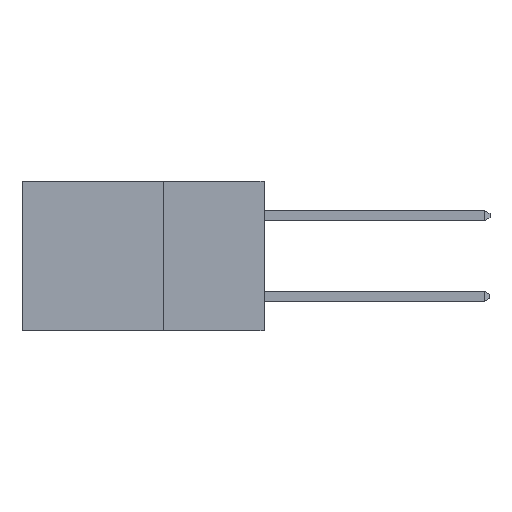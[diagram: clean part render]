
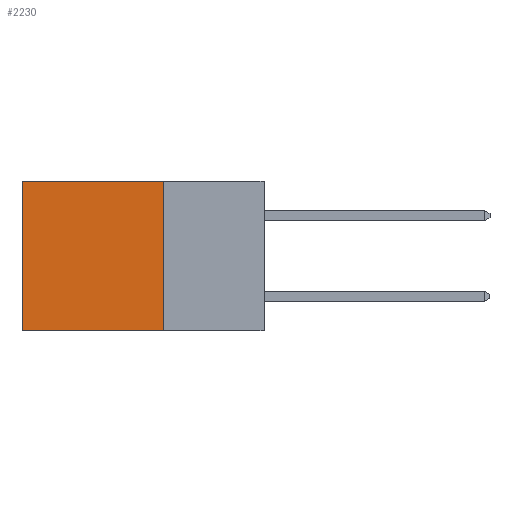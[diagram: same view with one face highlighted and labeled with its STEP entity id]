
A CAD part, left-side view. The second image highlights one B-rep face of the part: STEP entity #2230.
In plain terms, the highlighted planar face has unit normal (-1, 0, 0).
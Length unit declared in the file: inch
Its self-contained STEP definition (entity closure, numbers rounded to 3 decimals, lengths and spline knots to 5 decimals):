
#500 = EDGE_CURVE ( 'NONE', #7606, #8328, #4183, .T. ) ;
#1418 = ORIENTED_EDGE ( 'NONE', *, *, #4598, .T. ) ;
#1744 = DIRECTION ( 'NONE',  ( 0., 0., -1. ) ) ;
#1900 = DIRECTION ( 'NONE',  ( 0., 1., 0. ) ) ;
#1957 = VERTEX_POINT ( 'NONE', #8599 ) ;
#2120 = CARTESIAN_POINT ( 'NONE',  ( 0.2615, 0.25, 0. ) ) ;
#2121 = VERTEX_POINT ( 'NONE', #8444 ) ;
#2230 = ADVANCED_FACE ( 'NONE', ( #8394 ), #9213, .F. ) ;
#2244 = ORIENTED_EDGE ( 'NONE', *, *, #9056, .F. ) ;
#2339 = DIRECTION ( 'NONE',  ( 0., 0., -1. ) ) ;
#2359 = AXIS2_PLACEMENT_3D ( 'NONE', #9157, #2833, #9413 ) ;
#2518 = CARTESIAN_POINT ( 'NONE',  ( 0.2615, 0.25, -0.37 ) ) ;
#2833 = DIRECTION ( 'NONE',  ( 1., 0., 0. ) ) ;
#4054 = LINE ( 'NONE', #7241, #5499 ) ;
#4094 = LINE ( 'NONE', #6432, #5675 ) ;
#4183 = LINE ( 'NONE', #9747, #5618 ) ;
#4256 = ORIENTED_EDGE ( 'NONE', *, *, #5012, .F. ) ;
#4426 = EDGE_LOOP ( 'NONE', ( #1418, #4256, #2244, #9916 ) ) ;
#4598 = EDGE_CURVE ( 'NONE', #8328, #2121, #4054, .T. ) ;
#5012 = EDGE_CURVE ( 'NONE', #1957, #2121, #4094, .T. ) ;
#5127 = CARTESIAN_POINT ( 'NONE',  ( 0.2615, 0.6, 0. ) ) ;
#5499 = VECTOR ( 'NONE', #2339, 39.37008 ) ;
#5618 = VECTOR ( 'NONE', #1900, 39.37008 ) ;
#5675 = VECTOR ( 'NONE', #8727, 39.37008 ) ;
#6429 = LINE ( 'NONE', #2518, #7558 ) ;
#6432 = CARTESIAN_POINT ( 'NONE',  ( 0.2615, 0.25, -0.37 ) ) ;
#7241 = CARTESIAN_POINT ( 'NONE',  ( 0.2615, 0.6, -0.37 ) ) ;
#7558 = VECTOR ( 'NONE', #1744, 39.37008 ) ;
#7606 = VERTEX_POINT ( 'NONE', #2120 ) ;
#8328 = VERTEX_POINT ( 'NONE', #5127 ) ;
#8394 = FACE_OUTER_BOUND ( 'NONE', #4426, .T. ) ;
#8444 = CARTESIAN_POINT ( 'NONE',  ( 0.2615, 0.6, -0.37 ) ) ;
#8599 = CARTESIAN_POINT ( 'NONE',  ( 0.2615, 0.25, -0.37 ) ) ;
#8727 = DIRECTION ( 'NONE',  ( 0., 1., 0. ) ) ;
#9056 = EDGE_CURVE ( 'NONE', #7606, #1957, #6429, .T. ) ;
#9157 = CARTESIAN_POINT ( 'NONE',  ( 0.2615, 0.25, -0.37 ) ) ;
#9213 = PLANE ( 'NONE',  #2359 ) ;
#9413 = DIRECTION ( 'NONE',  ( 0., 0., -1. ) ) ;
#9747 = CARTESIAN_POINT ( 'NONE',  ( 0.2615, 0.25, 0. ) ) ;
#9916 = ORIENTED_EDGE ( 'NONE', *, *, #500, .T. ) ;
